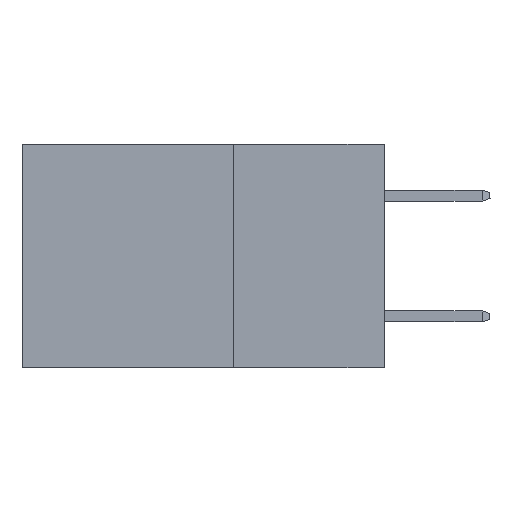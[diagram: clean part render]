
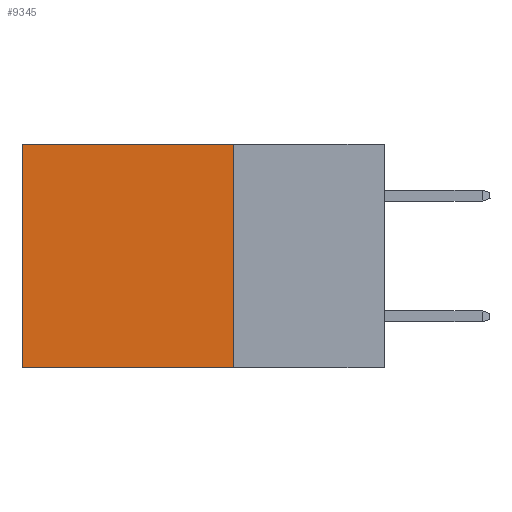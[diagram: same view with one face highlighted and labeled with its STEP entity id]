
A CAD part, left-side view. The second image highlights one B-rep face of the part: STEP entity #9345.
In plain terms, the highlighted planar face has unit normal (-1, 0, 0).
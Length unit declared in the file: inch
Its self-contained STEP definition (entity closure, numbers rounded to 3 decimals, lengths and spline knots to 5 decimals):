
#494 = DIRECTION ( 'NONE',  ( 0., 0., -1. ) ) ;
#960 = CARTESIAN_POINT ( 'NONE',  ( 0.298, 0.25, 0. ) ) ;
#2315 = CARTESIAN_POINT ( 'NONE',  ( 0.298, 0.6, -0.37 ) ) ;
#2448 = CARTESIAN_POINT ( 'NONE',  ( 0.298, 0.25, 0. ) ) ;
#2553 = VECTOR ( 'NONE', #13204, 39.37008 ) ;
#2556 = CARTESIAN_POINT ( 'NONE',  ( 0.298, 0.25, -0.37 ) ) ;
#2902 = DIRECTION ( 'NONE',  ( 0., 0., -1. ) ) ;
#3064 = DIRECTION ( 'NONE',  ( 0., 1., 0. ) ) ;
#3907 = VERTEX_POINT ( 'NONE', #10717 ) ;
#5132 = EDGE_CURVE ( 'NONE', #17132, #3907, #7839, .T. ) ;
#5349 = ORIENTED_EDGE ( 'NONE', *, *, #14780, .T. ) ;
#6528 = LINE ( 'NONE', #2556, #9952 ) ;
#6775 = VERTEX_POINT ( 'NONE', #12296 ) ;
#7839 = LINE ( 'NONE', #15728, #2553 ) ;
#8795 = EDGE_CURVE ( 'NONE', #17132, #6775, #15657, .T. ) ;
#9345 = ADVANCED_FACE ( 'NONE', ( #19883 ), #14088, .F. ) ;
#9952 = VECTOR ( 'NONE', #20369, 39.37008 ) ;
#10376 = VECTOR ( 'NONE', #3064, 39.37008 ) ;
#10427 = CARTESIAN_POINT ( 'NONE',  ( 0.298, 0.6, 0. ) ) ;
#10717 = CARTESIAN_POINT ( 'NONE',  ( 0.298, 0.25, -0.37 ) ) ;
#12296 = CARTESIAN_POINT ( 'NONE',  ( 0.298, 0.6, 0. ) ) ;
#12943 = DIRECTION ( 'NONE',  ( 1., 0., 0. ) ) ;
#13204 = DIRECTION ( 'NONE',  ( 0., 0., -1. ) ) ;
#13284 = CARTESIAN_POINT ( 'NONE',  ( 0.298, 0.25, 0. ) ) ;
#13413 = VECTOR ( 'NONE', #494, 39.37008 ) ;
#14088 = PLANE ( 'NONE',  #19424 ) ;
#14188 = ORIENTED_EDGE ( 'NONE', *, *, #8795, .T. ) ;
#14353 = ORIENTED_EDGE ( 'NONE', *, *, #5132, .F. ) ;
#14780 = EDGE_CURVE ( 'NONE', #6775, #15392, #23862, .T. ) ;
#15392 = VERTEX_POINT ( 'NONE', #2315 ) ;
#15657 = LINE ( 'NONE', #960, #10376 ) ;
#15728 = CARTESIAN_POINT ( 'NONE',  ( 0.298, 0.25, 0. ) ) ;
#17132 = VERTEX_POINT ( 'NONE', #2448 ) ;
#17780 = ORIENTED_EDGE ( 'NONE', *, *, #24063, .F. ) ;
#18802 = EDGE_LOOP ( 'NONE', ( #5349, #17780, #14353, #14188 ) ) ;
#19424 = AXIS2_PLACEMENT_3D ( 'NONE', #13284, #12943, #2902 ) ;
#19883 = FACE_OUTER_BOUND ( 'NONE', #18802, .T. ) ;
#20369 = DIRECTION ( 'NONE',  ( 0., 1., 0. ) ) ;
#23862 = LINE ( 'NONE', #10427, #13413 ) ;
#24063 = EDGE_CURVE ( 'NONE', #3907, #15392, #6528, .T. ) ;
